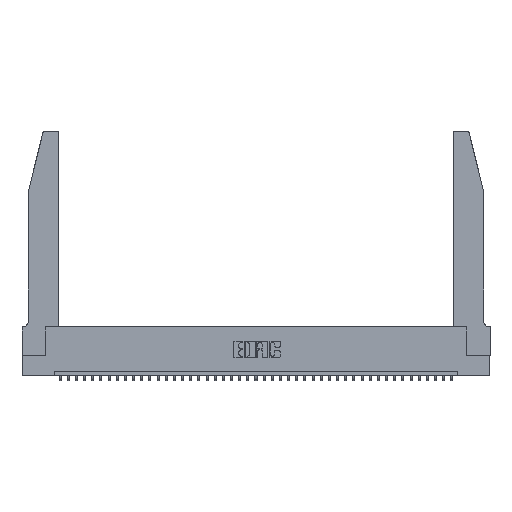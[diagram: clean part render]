
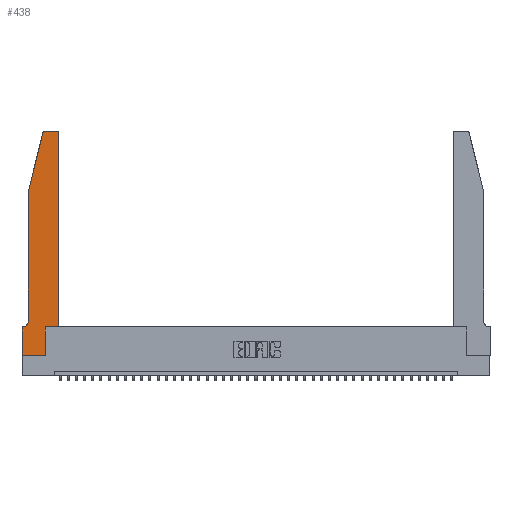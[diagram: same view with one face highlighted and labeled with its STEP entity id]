
A CAD part, top view. The second image highlights one B-rep face of the part: STEP entity #438.
In plain terms, the highlighted planar face has unit normal (0, 0, 1).
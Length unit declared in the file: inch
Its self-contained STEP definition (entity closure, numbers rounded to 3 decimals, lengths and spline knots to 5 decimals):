
#91 = CARTESIAN_POINT ( 'NONE',  ( 0.0055, 0.35, 0.37 ) ) ;
#309 = CIRCLE ( 'NONE', #24026, 0.03 ) ;
#319 = CARTESIAN_POINT ( 'NONE',  ( 0., 0., 0.37 ) ) ;
#438 = ADVANCED_FACE ( 'NONE', ( #32435 ), #34270, .T. ) ;
#475 = EDGE_CURVE ( 'NONE', #29165, #3902, #31029, .T. ) ;
#1066 = EDGE_CURVE ( 'NONE', #39246, #36294, #24136, .T. ) ;
#1080 = DIRECTION ( 'NONE',  ( 0., 0., 1. ) ) ;
#3115 = EDGE_CURVE ( 'NONE', #36885, #11961, #29851, .T. ) ;
#3156 = DIRECTION ( 'NONE',  ( 0., -1., 0. ) ) ;
#3243 = CARTESIAN_POINT ( 'NONE',  ( 0.4205, 2.72, 0.37 ) ) ;
#3253 = VERTEX_POINT ( 'NONE', #91 ) ;
#3510 = DIRECTION ( 'NONE',  ( 1., 0., 0. ) ) ;
#3902 = VERTEX_POINT ( 'NONE', #40462 ) ;
#4265 = CARTESIAN_POINT ( 'NONE',  ( 0.0755, 2., 0.37 ) ) ;
#4866 = EDGE_CURVE ( 'NONE', #3902, #24153, #5210, .T. ) ;
#5210 = LINE ( 'NONE', #29528, #28862 ) ;
#5507 = EDGE_LOOP ( 'NONE', ( #25554, #22210, #9505, #9655, #31432, #37944, #36182, #36521, #26913, #13245, #18593, #7446 ) ) ;
#5808 = DIRECTION ( 'NONE',  ( -1., 0., 0. ) ) ;
#5985 = CARTESIAN_POINT ( 'NONE',  ( 0.4505, 0.35, 0.37 ) ) ;
#6354 = DIRECTION ( 'NONE',  ( 1., 0., 0. ) ) ;
#6478 = CARTESIAN_POINT ( 'NONE',  ( 0., 0.35, 0.37 ) ) ;
#6856 = CARTESIAN_POINT ( 'NONE',  ( 0.2865, 0.35, 0.37 ) ) ;
#7161 = CARTESIAN_POINT ( 'NONE',  ( 0.284, 2.72, 0.37 ) ) ;
#7431 = AXIS2_PLACEMENT_3D ( 'NONE', #6478, #28283, #6354 ) ;
#7446 = ORIENTED_EDGE ( 'NONE', *, *, #15889, .T. ) ;
#7869 = CARTESIAN_POINT ( 'NONE',  ( 0.0755, 2., 0.37 ) ) ;
#8175 = CIRCLE ( 'NONE', #32715, 0.03 ) ;
#8205 = EDGE_CURVE ( 'NONE', #10062, #3253, #31100, .T. ) ;
#8595 = LINE ( 'NONE', #38786, #31645 ) ;
#8817 = EDGE_CURVE ( 'NONE', #26936, #20745, #16762, .T. ) ;
#9298 = EDGE_CURVE ( 'NONE', #3253, #18290, #29016, .T. ) ;
#9505 = ORIENTED_EDGE ( 'NONE', *, *, #8817, .T. ) ;
#9655 = ORIENTED_EDGE ( 'NONE', *, *, #10230, .T. ) ;
#9832 = VECTOR ( 'NONE', #40644, 39.37008 ) ;
#10062 = VERTEX_POINT ( 'NONE', #24476 ) ;
#10230 = EDGE_CURVE ( 'NONE', #20745, #10062, #21465, .T. ) ;
#10606 = DIRECTION ( 'NONE',  ( -0.239, -0.971, 0. ) ) ;
#10662 = DIRECTION ( 'NONE',  ( 0., 1., 0. ) ) ;
#11961 = VERTEX_POINT ( 'NONE', #32329 ) ;
#12749 = DIRECTION ( 'NONE',  ( 0., 0., 1. ) ) ;
#13033 = VECTOR ( 'NONE', #3156, 39.37008 ) ;
#13221 = CARTESIAN_POINT ( 'NONE',  ( 0.2865, 0.35, 0.37 ) ) ;
#13245 = ORIENTED_EDGE ( 'NONE', *, *, #475, .T. ) ;
#13384 = LINE ( 'NONE', #13221, #38440 ) ;
#13494 = DIRECTION ( 'NONE',  ( 0., 1., 0. ) ) ;
#13548 = CARTESIAN_POINT ( 'NONE',  ( 0.4205, 2.75, 0.37 ) ) ;
#14126 = EDGE_CURVE ( 'NONE', #11961, #26936, #309, .T. ) ;
#15107 = CARTESIAN_POINT ( 'NONE',  ( 0.25487, 2.72718, 0.37 ) ) ;
#15889 = EDGE_CURVE ( 'NONE', #24153, #36885, #8175, .T. ) ;
#15932 = DIRECTION ( 'NONE',  ( 1., 0., 0. ) ) ;
#16762 = LINE ( 'NONE', #4265, #19715 ) ;
#17577 = VECTOR ( 'NONE', #20497, 39.37008 ) ;
#18290 = VERTEX_POINT ( 'NONE', #20964 ) ;
#18593 = ORIENTED_EDGE ( 'NONE', *, *, #4866, .T. ) ;
#18878 = CARTESIAN_POINT ( 'NONE',  ( 0.0755, 2., 0.37 ) ) ;
#19715 = VECTOR ( 'NONE', #10606, 39.37008 ) ;
#20497 = DIRECTION ( 'NONE',  ( -1., 0., 0. ) ) ;
#20671 = VECTOR ( 'NONE', #5808, 39.37008 ) ;
#20709 = VECTOR ( 'NONE', #3510, 39.37008 ) ;
#20745 = VERTEX_POINT ( 'NONE', #7869 ) ;
#20964 = CARTESIAN_POINT ( 'NONE',  ( 0., 0.35, 0.37 ) ) ;
#21465 = LINE ( 'NONE', #18878, #13033 ) ;
#21517 = DIRECTION ( 'NONE',  ( -1., 0., 0. ) ) ;
#22210 = ORIENTED_EDGE ( 'NONE', *, *, #14126, .T. ) ;
#24026 = AXIS2_PLACEMENT_3D ( 'NONE', #7161, #1080, #30447 ) ;
#24136 = LINE ( 'NONE', #319, #20709 ) ;
#24153 = VERTEX_POINT ( 'NONE', #29493 ) ;
#24235 = CARTESIAN_POINT ( 'NONE',  ( 0.0755, 0.35, 0.37 ) ) ;
#24476 = CARTESIAN_POINT ( 'NONE',  ( 0.0755, 0.42, 0.37 ) ) ;
#25554 = ORIENTED_EDGE ( 'NONE', *, *, #3115, .T. ) ;
#26913 = ORIENTED_EDGE ( 'NONE', *, *, #27521, .T. ) ;
#26936 = VERTEX_POINT ( 'NONE', #15107 ) ;
#27521 = EDGE_CURVE ( 'NONE', #36294, #29165, #13384, .T. ) ;
#27717 = CARTESIAN_POINT ( 'NONE',  ( 0.0055, 0.42, 0.37 ) ) ;
#28283 = DIRECTION ( 'NONE',  ( 0., 0., 1. ) ) ;
#28862 = VECTOR ( 'NONE', #10662, 39.37008 ) ;
#29016 = LINE ( 'NONE', #24235, #20671 ) ;
#29165 = VERTEX_POINT ( 'NONE', #6856 ) ;
#29493 = CARTESIAN_POINT ( 'NONE',  ( 0.4505, 2.72, 0.37 ) ) ;
#29528 = CARTESIAN_POINT ( 'NONE',  ( 0.4505, 0.35, 0.37 ) ) ;
#29851 = LINE ( 'NONE', #36134, #17577 ) ;
#30407 = DIRECTION ( 'NONE',  ( 0., 0., -1. ) ) ;
#30447 = DIRECTION ( 'NONE',  ( 1., 0., 0. ) ) ;
#31029 = LINE ( 'NONE', #5985, #9832 ) ;
#31100 = CIRCLE ( 'NONE', #33631, 0.07 ) ;
#31432 = ORIENTED_EDGE ( 'NONE', *, *, #8205, .T. ) ;
#31645 = VECTOR ( 'NONE', #38637, 39.37008 ) ;
#31863 = CARTESIAN_POINT ( 'NONE',  ( 0.2865, 0., 0.37 ) ) ;
#32205 = EDGE_CURVE ( 'NONE', #18290, #39246, #8595, .T. ) ;
#32329 = CARTESIAN_POINT ( 'NONE',  ( 0.284, 2.75, 0.37 ) ) ;
#32435 = FACE_OUTER_BOUND ( 'NONE', #5507, .T. ) ;
#32715 = AXIS2_PLACEMENT_3D ( 'NONE', #3243, #12749, #15932 ) ;
#33631 = AXIS2_PLACEMENT_3D ( 'NONE', #27717, #30407, #21517 ) ;
#34270 = PLANE ( 'NONE',  #7431 ) ;
#36134 = CARTESIAN_POINT ( 'NONE',  ( 0.2605, 2.75, 0.37 ) ) ;
#36182 = ORIENTED_EDGE ( 'NONE', *, *, #32205, .T. ) ;
#36294 = VERTEX_POINT ( 'NONE', #31863 ) ;
#36521 = ORIENTED_EDGE ( 'NONE', *, *, #1066, .T. ) ;
#36885 = VERTEX_POINT ( 'NONE', #13548 ) ;
#37944 = ORIENTED_EDGE ( 'NONE', *, *, #9298, .T. ) ;
#38440 = VECTOR ( 'NONE', #13494, 39.37008 ) ;
#38527 = CARTESIAN_POINT ( 'NONE',  ( 0., 0., 0.37 ) ) ;
#38637 = DIRECTION ( 'NONE',  ( 0., -1., 0. ) ) ;
#38786 = CARTESIAN_POINT ( 'NONE',  ( 0., 0., 0.37 ) ) ;
#39246 = VERTEX_POINT ( 'NONE', #38527 ) ;
#40462 = CARTESIAN_POINT ( 'NONE',  ( 0.4505, 0.35, 0.37 ) ) ;
#40644 = DIRECTION ( 'NONE',  ( 1., 0., 0. ) ) ;
